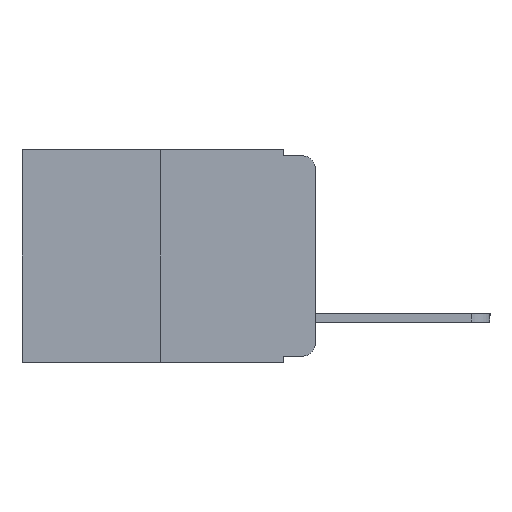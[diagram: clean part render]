
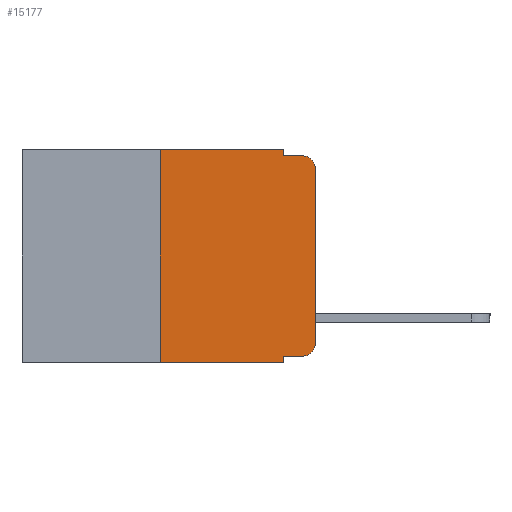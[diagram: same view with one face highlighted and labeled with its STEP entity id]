
A CAD part, left-side view. The second image highlights one B-rep face of the part: STEP entity #15177.
In plain terms, the highlighted planar face has unit normal (-1, 0, 0).
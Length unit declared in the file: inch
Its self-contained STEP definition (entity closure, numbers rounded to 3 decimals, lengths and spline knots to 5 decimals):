
#58 = LINE ( 'NONE', #19978, #12711 ) ;
#162 = EDGE_CURVE ( 'NONE', #13496, #1456, #58, .T. ) ;
#292 = CIRCLE ( 'NONE', #13779, 0.02 ) ;
#368 = ORIENTED_EDGE ( 'NONE', *, *, #5558, .T. ) ;
#402 = CARTESIAN_POINT ( 'NONE',  ( 0., 0.051, -0.333 ) ) ;
#509 = CARTESIAN_POINT ( 'NONE',  ( 0., 0.051, 0. ) ) ;
#761 = DIRECTION ( 'NONE',  ( 0., 0., 1. ) ) ;
#1328 = VECTOR ( 'NONE', #3943, 39.37008 ) ;
#1392 = CARTESIAN_POINT ( 'NONE',  ( 0., 0.473, 0. ) ) ;
#1456 = VERTEX_POINT ( 'NONE', #20662 ) ;
#1583 = DIRECTION ( 'NONE',  ( -1., 0., 0. ) ) ;
#2032 = LINE ( 'NONE', #12205, #10253 ) ;
#2037 = ORIENTED_EDGE ( 'NONE', *, *, #12062, .T. ) ;
#2386 = LINE ( 'NONE', #509, #1328 ) ;
#2472 = DIRECTION ( 'NONE',  ( 0., -1., 0. ) ) ;
#2574 = ORIENTED_EDGE ( 'NONE', *, *, #8899, .F. ) ;
#3436 = DIRECTION ( 'NONE',  ( 0., -1., 0. ) ) ;
#3943 = DIRECTION ( 'NONE',  ( 0., 0., -1. ) ) ;
#4192 = VERTEX_POINT ( 'NONE', #402 ) ;
#4466 = EDGE_CURVE ( 'NONE', #11361, #6054, #292, .T. ) ;
#4471 = VECTOR ( 'NONE', #12835, 39.37008 ) ;
#4675 = CARTESIAN_POINT ( 'NONE',  ( 0., 0.051, 0. ) ) ;
#4895 = ORIENTED_EDGE ( 'NONE', *, *, #4466, .T. ) ;
#5540 = AXIS2_PLACEMENT_3D ( 'NONE', #11395, #1583, #12987 ) ;
#5558 = EDGE_CURVE ( 'NONE', #4192, #11361, #19125, .T. ) ;
#5931 = CARTESIAN_POINT ( 'NONE',  ( 0., 0., -0.03 ) ) ;
#6054 = VERTEX_POINT ( 'NONE', #7691 ) ;
#6173 = FACE_OUTER_BOUND ( 'NONE', #15903, .T. ) ;
#6362 = DIRECTION ( 'NONE',  ( 0., 0., -1. ) ) ;
#6446 = DIRECTION ( 'NONE',  ( 1., 0., 0. ) ) ;
#6720 = EDGE_CURVE ( 'NONE', #4192, #1456, #11088, .T. ) ;
#7191 = CARTESIAN_POINT ( 'NONE',  ( 0., 0.051, 0. ) ) ;
#7381 = VERTEX_POINT ( 'NONE', #8712 ) ;
#7651 = VECTOR ( 'NONE', #761, 39.37008 ) ;
#7691 = CARTESIAN_POINT ( 'NONE',  ( 0., 0., -0.313 ) ) ;
#7806 = EDGE_CURVE ( 'NONE', #13496, #14673, #10282, .T. ) ;
#8361 = CARTESIAN_POINT ( 'NONE',  ( 0., 0.02, -0.01 ) ) ;
#8712 = CARTESIAN_POINT ( 'NONE',  ( 0., 0.051, -0.01 ) ) ;
#8899 = EDGE_CURVE ( 'NONE', #14827, #7381, #2386, .T. ) ;
#9082 = CARTESIAN_POINT ( 'NONE',  ( 0., 0., 0. ) ) ;
#9448 = AXIS2_PLACEMENT_3D ( 'NONE', #1392, #6446, #17477 ) ;
#9928 = EDGE_CURVE ( 'NONE', #7381, #15941, #16677, .T. ) ;
#10253 = VECTOR ( 'NONE', #19953, 39.37008 ) ;
#10282 = LINE ( 'NONE', #12840, #13974 ) ;
#11088 = LINE ( 'NONE', #4675, #18816 ) ;
#11294 = CARTESIAN_POINT ( 'NONE',  ( 0., 0.25, 0. ) ) ;
#11361 = VERTEX_POINT ( 'NONE', #12223 ) ;
#11390 = LINE ( 'NONE', #9082, #7651 ) ;
#11395 = CARTESIAN_POINT ( 'NONE',  ( 0., 0.02, -0.03 ) ) ;
#11771 = ORIENTED_EDGE ( 'NONE', *, *, #18156, .F. ) ;
#12062 = EDGE_CURVE ( 'NONE', #16505, #15941, #17234, .T. ) ;
#12205 = CARTESIAN_POINT ( 'NONE',  ( 0., 0.473, 0. ) ) ;
#12223 = CARTESIAN_POINT ( 'NONE',  ( 0., 0.02, -0.333 ) ) ;
#12233 = CARTESIAN_POINT ( 'NONE',  ( 0., 0.051, -0.333 ) ) ;
#12711 = VECTOR ( 'NONE', #3436, 39.37008 ) ;
#12835 = DIRECTION ( 'NONE',  ( 0., -1., 0. ) ) ;
#12840 = CARTESIAN_POINT ( 'NONE',  ( 0., 0.25, 0. ) ) ;
#12987 = DIRECTION ( 'NONE',  ( 0., 0., -1. ) ) ;
#13125 = EDGE_CURVE ( 'NONE', #6054, #16505, #11390, .T. ) ;
#13192 = CARTESIAN_POINT ( 'NONE',  ( 0., 0.25, -0.343 ) ) ;
#13238 = ORIENTED_EDGE ( 'NONE', *, *, #6720, .F. ) ;
#13496 = VERTEX_POINT ( 'NONE', #13192 ) ;
#13779 = AXIS2_PLACEMENT_3D ( 'NONE', #13888, #13863, #19496 ) ;
#13863 = DIRECTION ( 'NONE',  ( -1., 0., 0. ) ) ;
#13888 = CARTESIAN_POINT ( 'NONE',  ( 0., 0.02, -0.313 ) ) ;
#13974 = VECTOR ( 'NONE', #20511, 39.37008 ) ;
#14673 = VERTEX_POINT ( 'NONE', #11294 ) ;
#14827 = VERTEX_POINT ( 'NONE', #7191 ) ;
#14932 = ORIENTED_EDGE ( 'NONE', *, *, #9928, .F. ) ;
#15068 = VECTOR ( 'NONE', #2472, 39.37008 ) ;
#15177 = ADVANCED_FACE ( 'NONE', ( #6173 ), #15928, .F. ) ;
#15903 = EDGE_LOOP ( 'NONE', ( #18522, #2037, #14932, #2574, #11771, #15909, #20470, #13238, #368, #4895 ) ) ;
#15909 = ORIENTED_EDGE ( 'NONE', *, *, #7806, .F. ) ;
#15928 = PLANE ( 'NONE',  #9448 ) ;
#15941 = VERTEX_POINT ( 'NONE', #8361 ) ;
#16505 = VERTEX_POINT ( 'NONE', #5931 ) ;
#16677 = LINE ( 'NONE', #17428, #4471 ) ;
#17234 = CIRCLE ( 'NONE', #5540, 0.02 ) ;
#17428 = CARTESIAN_POINT ( 'NONE',  ( 0., 0.051, -0.01 ) ) ;
#17477 = DIRECTION ( 'NONE',  ( 0., 0., -1. ) ) ;
#18156 = EDGE_CURVE ( 'NONE', #14673, #14827, #2032, .T. ) ;
#18522 = ORIENTED_EDGE ( 'NONE', *, *, #13125, .T. ) ;
#18816 = VECTOR ( 'NONE', #6362, 39.37008 ) ;
#19125 = LINE ( 'NONE', #12233, #15068 ) ;
#19496 = DIRECTION ( 'NONE',  ( 0., 0., -1. ) ) ;
#19953 = DIRECTION ( 'NONE',  ( 0., -1., 0. ) ) ;
#19978 = CARTESIAN_POINT ( 'NONE',  ( 0., 0.473, -0.343 ) ) ;
#20470 = ORIENTED_EDGE ( 'NONE', *, *, #162, .T. ) ;
#20511 = DIRECTION ( 'NONE',  ( 0., 0., 1. ) ) ;
#20662 = CARTESIAN_POINT ( 'NONE',  ( 0., 0.051, -0.343 ) ) ;
